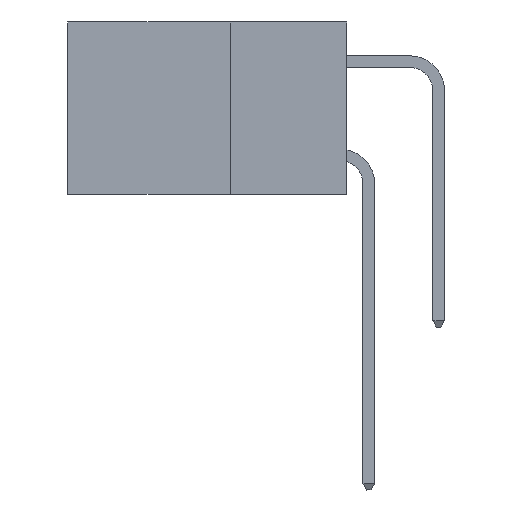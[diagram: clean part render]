
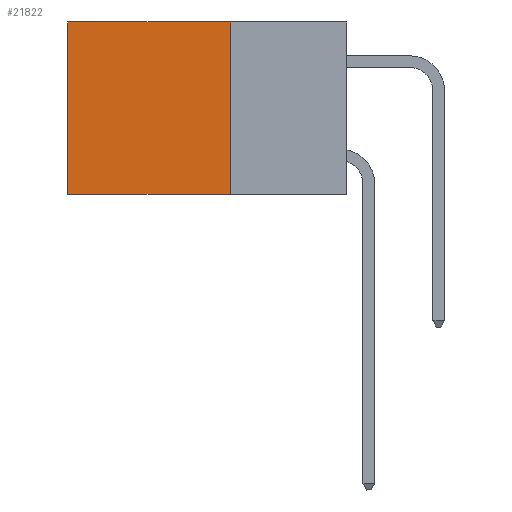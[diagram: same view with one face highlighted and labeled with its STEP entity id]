
A CAD part, left-side view. The second image highlights one B-rep face of the part: STEP entity #21822.
In plain terms, the highlighted planar face has unit normal (-1, 0, 0).
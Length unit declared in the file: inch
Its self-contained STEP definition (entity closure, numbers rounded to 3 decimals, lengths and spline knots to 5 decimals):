
#6 = ORIENTED_EDGE ( 'NONE', *, *, #11655, .F. ) ;
#140 = CARTESIAN_POINT ( 'NONE',  ( 0.2875, 0.25, -0.37 ) ) ;
#1185 = VERTEX_POINT ( 'NONE', #21762 ) ;
#3236 = ORIENTED_EDGE ( 'NONE', *, *, #24377, .F. ) ;
#3792 = DIRECTION ( 'NONE',  ( 1., 0., 0. ) ) ;
#8456 = CARTESIAN_POINT ( 'NONE',  ( 0.2875, 0.25, 0. ) ) ;
#11338 = EDGE_CURVE ( 'NONE', #27954, #1185, #17046, .T. ) ;
#11655 = EDGE_CURVE ( 'NONE', #15854, #23996, #18936, .T. ) ;
#13467 = AXIS2_PLACEMENT_3D ( 'NONE', #17961, #3792, #30378 ) ;
#14163 = CARTESIAN_POINT ( 'NONE',  ( 0.2875, 0.25, -0.37 ) ) ;
#15854 = VERTEX_POINT ( 'NONE', #8456 ) ;
#17046 = LINE ( 'NONE', #27612, #28374 ) ;
#17414 = CARTESIAN_POINT ( 'NONE',  ( 0.2875, 0.25, 0. ) ) ;
#17807 = DIRECTION ( 'NONE',  ( 0., 0., -1. ) ) ;
#17828 = ORIENTED_EDGE ( 'NONE', *, *, #11338, .T. ) ;
#17961 = CARTESIAN_POINT ( 'NONE',  ( 0.2875, 0.25, 0. ) ) ;
#18936 = LINE ( 'NONE', #23710, #27228 ) ;
#21071 = EDGE_LOOP ( 'NONE', ( #17828, #3236, #6, #25896 ) ) ;
#21335 = DIRECTION ( 'NONE',  ( 0., 1., 0. ) ) ;
#21762 = CARTESIAN_POINT ( 'NONE',  ( 0.2875, 0.6, -0.37 ) ) ;
#21822 = ADVANCED_FACE ( 'NONE', ( #26097 ), #30061, .F. ) ;
#23710 = CARTESIAN_POINT ( 'NONE',  ( 0.2875, 0.25, 0. ) ) ;
#23996 = VERTEX_POINT ( 'NONE', #140 ) ;
#24377 = EDGE_CURVE ( 'NONE', #23996, #1185, #29885, .T. ) ;
#24668 = VECTOR ( 'NONE', #24731, 39.37008 ) ;
#24731 = DIRECTION ( 'NONE',  ( 0., 1., 0. ) ) ;
#25896 = ORIENTED_EDGE ( 'NONE', *, *, #29958, .T. ) ;
#26097 = FACE_OUTER_BOUND ( 'NONE', #21071, .T. ) ;
#27054 = CARTESIAN_POINT ( 'NONE',  ( 0.2875, 0.6, 0. ) ) ;
#27182 = VECTOR ( 'NONE', #21335, 39.37008 ) ;
#27228 = VECTOR ( 'NONE', #31383, 39.37008 ) ;
#27612 = CARTESIAN_POINT ( 'NONE',  ( 0.2875, 0.6, 0. ) ) ;
#27954 = VERTEX_POINT ( 'NONE', #27054 ) ;
#28374 = VECTOR ( 'NONE', #17807, 39.37008 ) ;
#29885 = LINE ( 'NONE', #14163, #27182 ) ;
#29958 = EDGE_CURVE ( 'NONE', #15854, #27954, #31144, .T. ) ;
#30061 = PLANE ( 'NONE',  #13467 ) ;
#30378 = DIRECTION ( 'NONE',  ( 0., 0., -1. ) ) ;
#31144 = LINE ( 'NONE', #17414, #24668 ) ;
#31383 = DIRECTION ( 'NONE',  ( 0., 0., -1. ) ) ;
